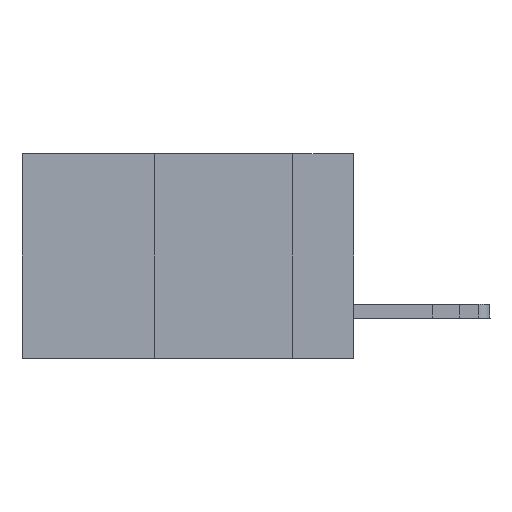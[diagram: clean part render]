
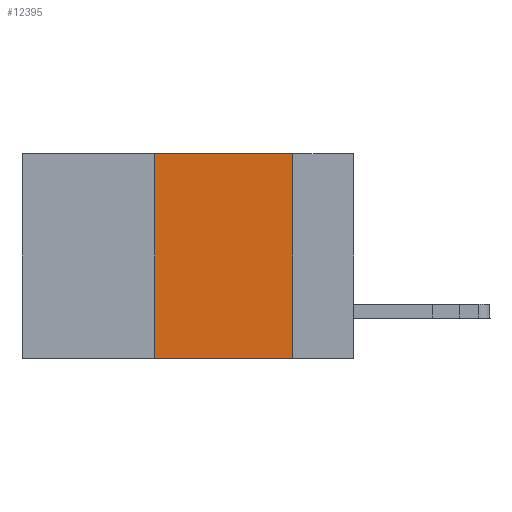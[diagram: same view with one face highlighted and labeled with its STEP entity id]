
A CAD part, left-side view. The second image highlights one B-rep face of the part: STEP entity #12395.
In plain terms, the highlighted planar face has unit normal (-1, 0, 0).
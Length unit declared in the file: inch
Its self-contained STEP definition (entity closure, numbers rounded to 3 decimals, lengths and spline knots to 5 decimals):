
#1207 = CARTESIAN_POINT ( 'NONE',  ( 0., 0.36, 0. ) ) ;
#2435 = EDGE_CURVE ( 'NONE', #18769, #11026, #11199, .T. ) ;
#2765 = CARTESIAN_POINT ( 'NONE',  ( 0., 0.11, 0. ) ) ;
#2865 = VECTOR ( 'NONE', #14073, 39.37008 ) ;
#2869 = CARTESIAN_POINT ( 'NONE',  ( 0., 0.6, 0. ) ) ;
#3502 = DIRECTION ( 'NONE',  ( 0., 0., -1. ) ) ;
#3961 = VERTEX_POINT ( 'NONE', #2765 ) ;
#4146 = CARTESIAN_POINT ( 'NONE',  ( 0., 0.11, -0.37 ) ) ;
#4432 = DIRECTION ( 'NONE',  ( 1., 0., 0. ) ) ;
#5346 = EDGE_LOOP ( 'NONE', ( #8646, #10772, #19590, #12875 ) ) ;
#6936 = FACE_OUTER_BOUND ( 'NONE', #5346, .T. ) ;
#7240 = DIRECTION ( 'NONE',  ( 0., 0., 1. ) ) ;
#8646 = ORIENTED_EDGE ( 'NONE', *, *, #10130, .F. ) ;
#8804 = CARTESIAN_POINT ( 'NONE',  ( 0., 0.36, 0. ) ) ;
#9940 = DIRECTION ( 'NONE',  ( 0., -1., 0. ) ) ;
#10130 = EDGE_CURVE ( 'NONE', #3961, #11026, #13817, .T. ) ;
#10772 = ORIENTED_EDGE ( 'NONE', *, *, #15194, .F. ) ;
#11026 = VERTEX_POINT ( 'NONE', #4146 ) ;
#11199 = LINE ( 'NONE', #12502, #2865 ) ;
#11306 = CARTESIAN_POINT ( 'NONE',  ( 0., 0.11, 0. ) ) ;
#11349 = AXIS2_PLACEMENT_3D ( 'NONE', #2869, #4432, #15270 ) ;
#11429 = LINE ( 'NONE', #8804, #18947 ) ;
#12395 = ADVANCED_FACE ( 'NONE', ( #6936 ), #13748, .F. ) ;
#12502 = CARTESIAN_POINT ( 'NONE',  ( 0., 0.6, -0.37 ) ) ;
#12875 = ORIENTED_EDGE ( 'NONE', *, *, #2435, .T. ) ;
#13748 = PLANE ( 'NONE',  #11349 ) ;
#13817 = LINE ( 'NONE', #11306, #16384 ) ;
#14073 = DIRECTION ( 'NONE',  ( 0., -1., 0. ) ) ;
#14160 = LINE ( 'NONE', #19034, #18591 ) ;
#14863 = CARTESIAN_POINT ( 'NONE',  ( 0., 0.36, -0.37 ) ) ;
#15194 = EDGE_CURVE ( 'NONE', #18885, #3961, #14160, .T. ) ;
#15270 = DIRECTION ( 'NONE',  ( 0., 0., -1. ) ) ;
#16384 = VECTOR ( 'NONE', #3502, 39.37008 ) ;
#18265 = EDGE_CURVE ( 'NONE', #18769, #18885, #11429, .T. ) ;
#18591 = VECTOR ( 'NONE', #9940, 39.37008 ) ;
#18769 = VERTEX_POINT ( 'NONE', #14863 ) ;
#18885 = VERTEX_POINT ( 'NONE', #1207 ) ;
#18947 = VECTOR ( 'NONE', #7240, 39.37008 ) ;
#19034 = CARTESIAN_POINT ( 'NONE',  ( 0., 0.6, 0. ) ) ;
#19590 = ORIENTED_EDGE ( 'NONE', *, *, #18265, .F. ) ;
